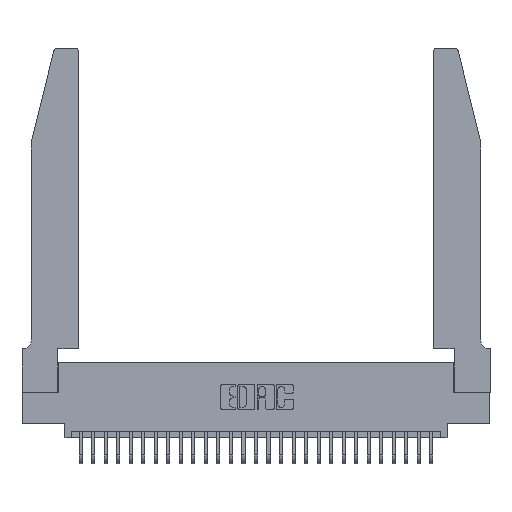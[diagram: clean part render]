
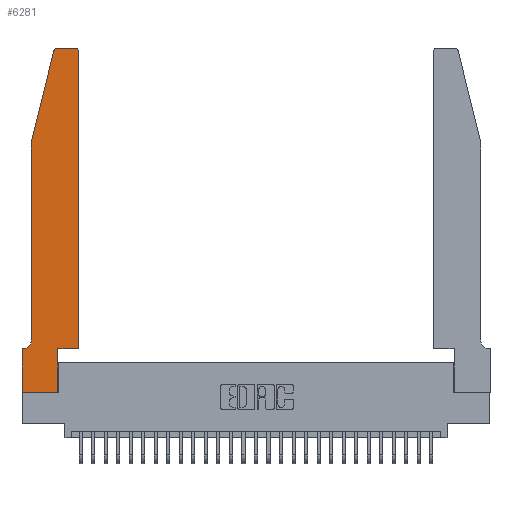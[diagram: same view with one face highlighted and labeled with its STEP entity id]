
A CAD part, top view. The second image highlights one B-rep face of the part: STEP entity #6281.
In plain terms, the highlighted planar face has unit normal (0, 0, 1).
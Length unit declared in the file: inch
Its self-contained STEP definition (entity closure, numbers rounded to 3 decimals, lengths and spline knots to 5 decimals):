
#25 = VERTEX_POINT ( 'NONE', #5316 ) ;
#115 = VERTEX_POINT ( 'NONE', #24493 ) ;
#458 = EDGE_CURVE ( 'NONE', #14339, #22890, #21997, .T. ) ;
#805 = CARTESIAN_POINT ( 'NONE',  ( 0.0755, 0.35, 0.37 ) ) ;
#1402 = LINE ( 'NONE', #22051, #4763 ) ;
#1533 = VECTOR ( 'NONE', #26241, 39.37008 ) ;
#1961 = CARTESIAN_POINT ( 'NONE',  ( 0., 0.35, 0.37 ) ) ;
#2977 = CIRCLE ( 'NONE', #11290, 0.07 ) ;
#3005 = DIRECTION ( 'NONE',  ( 1., 0., 0. ) ) ;
#3006 = DIRECTION ( 'NONE',  ( 0., -1., 0. ) ) ;
#3022 = DIRECTION ( 'NONE',  ( -1., 0., 0. ) ) ;
#4018 = ORIENTED_EDGE ( 'NONE', *, *, #27573, .T. ) ;
#4274 = PLANE ( 'NONE',  #29217 ) ;
#4548 = CARTESIAN_POINT ( 'NONE',  ( 0.4505, 0.35, 0.37 ) ) ;
#4763 = VECTOR ( 'NONE', #3006, 39.37008 ) ;
#5316 = CARTESIAN_POINT ( 'NONE',  ( 0.4505, 0.35, 0.37 ) ) ;
#5378 = ORIENTED_EDGE ( 'NONE', *, *, #25345, .T. ) ;
#5565 = CARTESIAN_POINT ( 'NONE',  ( 0.0055, 0.35, 0.37 ) ) ;
#6001 = CIRCLE ( 'NONE', #31077, 0.03 ) ;
#6281 = ADVANCED_FACE ( 'NONE', ( #19326 ), #4274, .T. ) ;
#6380 = CARTESIAN_POINT ( 'NONE',  ( 0.2865, 0.35, 0.37 ) ) ;
#6422 = LINE ( 'NONE', #18215, #10193 ) ;
#6617 = DIRECTION ( 'NONE',  ( 0., 1., 0. ) ) ;
#6697 = DIRECTION ( 'NONE',  ( 1., 0., 0. ) ) ;
#7314 = VECTOR ( 'NONE', #27807, 39.37008 ) ;
#7776 = CARTESIAN_POINT ( 'NONE',  ( 0.2865, 0.35, 0.37 ) ) ;
#8392 = VERTEX_POINT ( 'NONE', #30306 ) ;
#8721 = CARTESIAN_POINT ( 'NONE',  ( 0.2865, 0., 0.37 ) ) ;
#8967 = CARTESIAN_POINT ( 'NONE',  ( 0., 0., 0.37 ) ) ;
#8988 = VERTEX_POINT ( 'NONE', #1961 ) ;
#9118 = VECTOR ( 'NONE', #3022, 39.37008 ) ;
#9331 = DIRECTION ( 'NONE',  ( -1., 0., 0. ) ) ;
#9506 = LINE ( 'NONE', #26887, #9118 ) ;
#10193 = VECTOR ( 'NONE', #6617, 39.37008 ) ;
#11140 = EDGE_CURVE ( 'NONE', #115, #14339, #28246, .T. ) ;
#11290 = AXIS2_PLACEMENT_3D ( 'NONE', #23672, #16256, #9331 ) ;
#11519 = VERTEX_POINT ( 'NONE', #5565 ) ;
#11576 = CARTESIAN_POINT ( 'NONE',  ( 0., 0., 0.37 ) ) ;
#11671 = CARTESIAN_POINT ( 'NONE',  ( 0.4505, 2.72, 0.37 ) ) ;
#11704 = ORIENTED_EDGE ( 'NONE', *, *, #22276, .T. ) ;
#13357 = LINE ( 'NONE', #6380, #13737 ) ;
#13737 = VECTOR ( 'NONE', #27765, 39.37008 ) ;
#13759 = DIRECTION ( 'NONE',  ( 0., 0., 1. ) ) ;
#14339 = VERTEX_POINT ( 'NONE', #22610 ) ;
#14830 = LINE ( 'NONE', #8967, #7314 ) ;
#14866 = AXIS2_PLACEMENT_3D ( 'NONE', #20936, #13759, #6697 ) ;
#15292 = DIRECTION ( 'NONE',  ( 0., 0., 1. ) ) ;
#15503 = ORIENTED_EDGE ( 'NONE', *, *, #30840, .T. ) ;
#15526 = LINE ( 'NONE', #17185, #25670 ) ;
#16256 = DIRECTION ( 'NONE',  ( 0., 0., -1. ) ) ;
#16263 = ORIENTED_EDGE ( 'NONE', *, *, #458, .T. ) ;
#16809 = VERTEX_POINT ( 'NONE', #8721 ) ;
#17147 = ORIENTED_EDGE ( 'NONE', *, *, #17826, .T. ) ;
#17185 = CARTESIAN_POINT ( 'NONE',  ( 0., 0., 0.37 ) ) ;
#17288 = DIRECTION ( 'NONE',  ( 0., -1., 0. ) ) ;
#17627 = CARTESIAN_POINT ( 'NONE',  ( 0.0755, 2., 0.37 ) ) ;
#17826 = EDGE_CURVE ( 'NONE', #27930, #16809, #14830, .T. ) ;
#18215 = CARTESIAN_POINT ( 'NONE',  ( 0.4505, 0.35, 0.37 ) ) ;
#18311 = EDGE_CURVE ( 'NONE', #11519, #8988, #27526, .T. ) ;
#18333 = EDGE_LOOP ( 'NONE', ( #28305, #20924, #16263, #5378, #23184, #30354, #4018, #17147, #15503, #11704, #28553, #19148 ) ) ;
#19081 = EDGE_CURVE ( 'NONE', #20988, #115, #9506, .T. ) ;
#19148 = ORIENTED_EDGE ( 'NONE', *, *, #20360, .T. ) ;
#19326 = FACE_OUTER_BOUND ( 'NONE', #18333, .T. ) ;
#19877 = EDGE_CURVE ( 'NONE', #25, #20319, #6422, .T. ) ;
#20319 = VERTEX_POINT ( 'NONE', #11671 ) ;
#20360 = EDGE_CURVE ( 'NONE', #20319, #20988, #6001, .T. ) ;
#20505 = VECTOR ( 'NONE', #30669, 39.37008 ) ;
#20924 = ORIENTED_EDGE ( 'NONE', *, *, #11140, .T. ) ;
#20936 = CARTESIAN_POINT ( 'NONE',  ( 0.284, 2.72, 0.37 ) ) ;
#20988 = VERTEX_POINT ( 'NONE', #28767 ) ;
#21871 = VECTOR ( 'NONE', #29322, 39.37008 ) ;
#21997 = LINE ( 'NONE', #28354, #20505 ) ;
#22051 = CARTESIAN_POINT ( 'NONE',  ( 0.0755, 2., 0.37 ) ) ;
#22276 = EDGE_CURVE ( 'NONE', #25684, #25, #25558, .T. ) ;
#22480 = CARTESIAN_POINT ( 'NONE',  ( 0.4205, 2.72, 0.37 ) ) ;
#22610 = CARTESIAN_POINT ( 'NONE',  ( 0.25487, 2.72718, 0.37 ) ) ;
#22890 = VERTEX_POINT ( 'NONE', #17627 ) ;
#23184 = ORIENTED_EDGE ( 'NONE', *, *, #23777, .T. ) ;
#23672 = CARTESIAN_POINT ( 'NONE',  ( 0.0055, 0.42, 0.37 ) ) ;
#23777 = EDGE_CURVE ( 'NONE', #8392, #11519, #2977, .T. ) ;
#24493 = CARTESIAN_POINT ( 'NONE',  ( 0.284, 2.75, 0.37 ) ) ;
#25345 = EDGE_CURVE ( 'NONE', #22890, #8392, #1402, .T. ) ;
#25558 = LINE ( 'NONE', #4548, #1533 ) ;
#25670 = VECTOR ( 'NONE', #17288, 39.37008 ) ;
#25684 = VERTEX_POINT ( 'NONE', #7776 ) ;
#25694 = CARTESIAN_POINT ( 'NONE',  ( 0., 0.35, 0.37 ) ) ;
#26241 = DIRECTION ( 'NONE',  ( 1., 0., 0. ) ) ;
#26887 = CARTESIAN_POINT ( 'NONE',  ( 0.2605, 2.75, 0.37 ) ) ;
#27526 = LINE ( 'NONE', #805, #21871 ) ;
#27573 = EDGE_CURVE ( 'NONE', #8988, #27930, #15526, .T. ) ;
#27765 = DIRECTION ( 'NONE',  ( 0., 1., 0. ) ) ;
#27807 = DIRECTION ( 'NONE',  ( 1., 0., 0. ) ) ;
#27930 = VERTEX_POINT ( 'NONE', #11576 ) ;
#27966 = DIRECTION ( 'NONE',  ( 1., 0., 0. ) ) ;
#28246 = CIRCLE ( 'NONE', #14866, 0.03 ) ;
#28305 = ORIENTED_EDGE ( 'NONE', *, *, #19081, .T. ) ;
#28354 = CARTESIAN_POINT ( 'NONE',  ( 0.0755, 2., 0.37 ) ) ;
#28553 = ORIENTED_EDGE ( 'NONE', *, *, #19877, .T. ) ;
#28767 = CARTESIAN_POINT ( 'NONE',  ( 0.4205, 2.75, 0.37 ) ) ;
#29217 = AXIS2_PLACEMENT_3D ( 'NONE', #25694, #30285, #27966 ) ;
#29322 = DIRECTION ( 'NONE',  ( -1., 0., 0. ) ) ;
#30285 = DIRECTION ( 'NONE',  ( 0., 0., 1. ) ) ;
#30306 = CARTESIAN_POINT ( 'NONE',  ( 0.0755, 0.42, 0.37 ) ) ;
#30354 = ORIENTED_EDGE ( 'NONE', *, *, #18311, .T. ) ;
#30669 = DIRECTION ( 'NONE',  ( -0.239, -0.971, 0. ) ) ;
#30840 = EDGE_CURVE ( 'NONE', #16809, #25684, #13357, .T. ) ;
#31077 = AXIS2_PLACEMENT_3D ( 'NONE', #22480, #15292, #3005 ) ;
